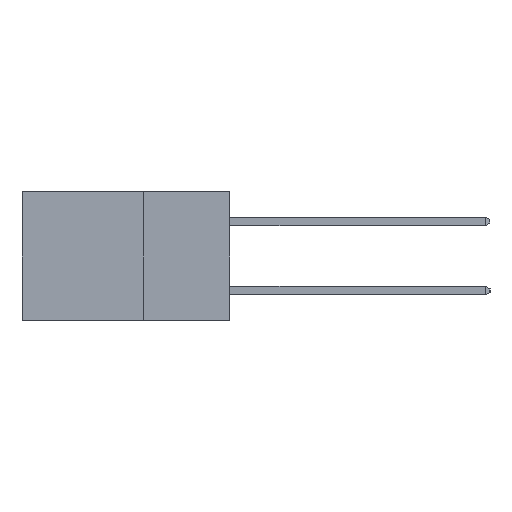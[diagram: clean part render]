
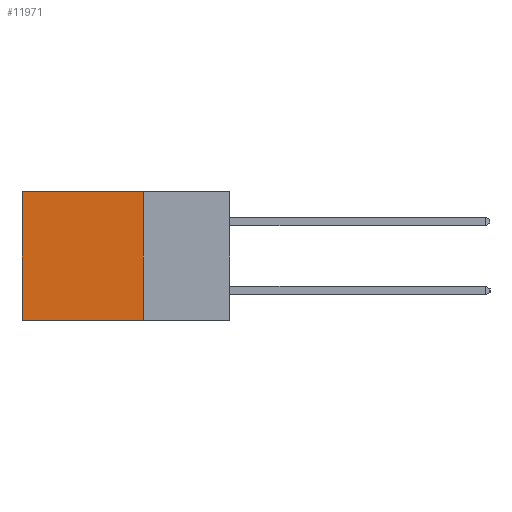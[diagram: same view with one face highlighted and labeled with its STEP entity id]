
A CAD part, left-side view. The second image highlights one B-rep face of the part: STEP entity #11971.
In plain terms, the highlighted planar face has unit normal (-1, 0, 0).
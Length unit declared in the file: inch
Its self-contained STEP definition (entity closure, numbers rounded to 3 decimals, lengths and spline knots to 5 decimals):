
#265 = CARTESIAN_POINT ( 'NONE',  ( 0.2615, 0.6, 0. ) ) ;
#899 = VECTOR ( 'NONE', #11677, 39.37008 ) ;
#2799 = EDGE_LOOP ( 'NONE', ( #10720, #14603, #16035, #12402 ) ) ;
#3296 = AXIS2_PLACEMENT_3D ( 'NONE', #4551, #16393, #7544 ) ;
#3799 = FACE_OUTER_BOUND ( 'NONE', #2799, .T. ) ;
#4315 = VERTEX_POINT ( 'NONE', #10122 ) ;
#4551 = CARTESIAN_POINT ( 'NONE',  ( 0.2615, 0.25, -0.37 ) ) ;
#5397 = LINE ( 'NONE', #7662, #16736 ) ;
#7182 = CARTESIAN_POINT ( 'NONE',  ( 0.2615, 0.25, -0.37 ) ) ;
#7544 = DIRECTION ( 'NONE',  ( 0., 0., -1. ) ) ;
#7662 = CARTESIAN_POINT ( 'NONE',  ( 0.2615, 0.6, -0.37 ) ) ;
#8208 = LINE ( 'NONE', #11936, #12162 ) ;
#8460 = EDGE_CURVE ( 'NONE', #16860, #12171, #10475, .T. ) ;
#9138 = DIRECTION ( 'NONE',  ( 0., 0., -1. ) ) ;
#10122 = CARTESIAN_POINT ( 'NONE',  ( 0.2615, 0.25, 0. ) ) ;
#10475 = LINE ( 'NONE', #7182, #17855 ) ;
#10720 = ORIENTED_EDGE ( 'NONE', *, *, #18654, .T. ) ;
#11620 = CARTESIAN_POINT ( 'NONE',  ( 0.2615, 0.25, -0.37 ) ) ;
#11677 = DIRECTION ( 'NONE',  ( 0., 1., 0. ) ) ;
#11936 = CARTESIAN_POINT ( 'NONE',  ( 0.2615, 0.25, -0.37 ) ) ;
#11963 = EDGE_CURVE ( 'NONE', #4315, #16860, #8208, .T. ) ;
#11971 = ADVANCED_FACE ( 'NONE', ( #3799 ), #14916, .F. ) ;
#12162 = VECTOR ( 'NONE', #13413, 39.37008 ) ;
#12171 = VERTEX_POINT ( 'NONE', #12588 ) ;
#12402 = ORIENTED_EDGE ( 'NONE', *, *, #14933, .T. ) ;
#12588 = CARTESIAN_POINT ( 'NONE',  ( 0.2615, 0.6, -0.37 ) ) ;
#13050 = DIRECTION ( 'NONE',  ( 0., 1., 0. ) ) ;
#13413 = DIRECTION ( 'NONE',  ( 0., 0., -1. ) ) ;
#14603 = ORIENTED_EDGE ( 'NONE', *, *, #8460, .F. ) ;
#14916 = PLANE ( 'NONE',  #3296 ) ;
#14933 = EDGE_CURVE ( 'NONE', #4315, #17977, #16201, .T. ) ;
#16035 = ORIENTED_EDGE ( 'NONE', *, *, #11963, .F. ) ;
#16201 = LINE ( 'NONE', #18999, #899 ) ;
#16393 = DIRECTION ( 'NONE',  ( 1., 0., 0. ) ) ;
#16736 = VECTOR ( 'NONE', #9138, 39.37008 ) ;
#16860 = VERTEX_POINT ( 'NONE', #11620 ) ;
#17855 = VECTOR ( 'NONE', #13050, 39.37008 ) ;
#17977 = VERTEX_POINT ( 'NONE', #265 ) ;
#18654 = EDGE_CURVE ( 'NONE', #17977, #12171, #5397, .T. ) ;
#18999 = CARTESIAN_POINT ( 'NONE',  ( 0.2615, 0.25, 0. ) ) ;
